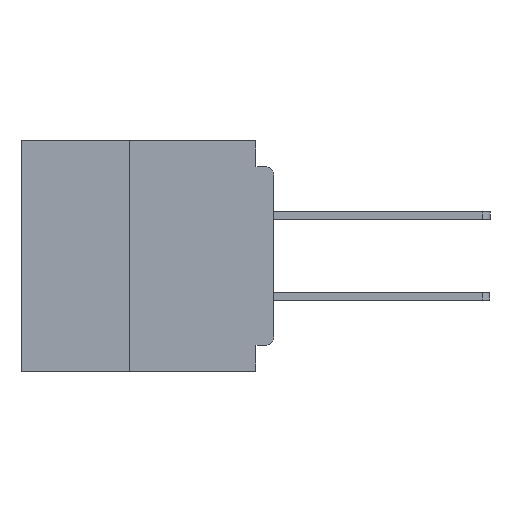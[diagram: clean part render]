
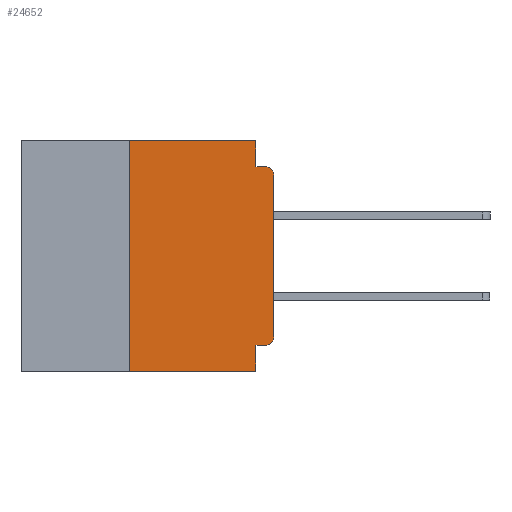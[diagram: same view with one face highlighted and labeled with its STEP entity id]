
A CAD part, left-side view. The second image highlights one B-rep face of the part: STEP entity #24652.
In plain terms, the highlighted planar face has unit normal (-1, 0, 0).
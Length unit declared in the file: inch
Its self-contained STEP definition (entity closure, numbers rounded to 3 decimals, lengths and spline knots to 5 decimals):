
#246 = DIRECTION ( 'NONE',  ( 1., 0., 0. ) ) ;
#389 = VERTEX_POINT ( 'NONE', #29512 ) ;
#532 = DIRECTION ( 'NONE',  ( 0., -1., 0. ) ) ;
#981 = VECTOR ( 'NONE', #20700, 39.37008 ) ;
#1316 = EDGE_CURVE ( 'NONE', #37058, #41313, #4289, .T. ) ;
#1412 = CIRCLE ( 'NONE', #5003, 0.015 ) ;
#1536 = EDGE_CURVE ( 'NONE', #41313, #11030, #31400, .T. ) ;
#1601 = DIRECTION ( 'NONE',  ( 0., -1., 0. ) ) ;
#1715 = ORIENTED_EDGE ( 'NONE', *, *, #9391, .T. ) ;
#2021 = EDGE_CURVE ( 'NONE', #21195, #37058, #12373, .T. ) ;
#3536 = CARTESIAN_POINT ( 'NONE',  ( 0., 0., -0.34 ) ) ;
#3734 = VECTOR ( 'NONE', #35093, 39.37008 ) ;
#3756 = CARTESIAN_POINT ( 'NONE',  ( 0., 0.437, 0. ) ) ;
#4183 = CARTESIAN_POINT ( 'NONE',  ( 0., 0.031, 0. ) ) ;
#4289 = LINE ( 'NONE', #3756, #20391 ) ;
#4397 = ORIENTED_EDGE ( 'NONE', *, *, #21143, .F. ) ;
#4438 = ORIENTED_EDGE ( 'NONE', *, *, #1536, .F. ) ;
#4540 = LINE ( 'NONE', #16035, #37647 ) ;
#5003 = AXIS2_PLACEMENT_3D ( 'NONE', #25646, #6422, #28865 ) ;
#5277 = EDGE_CURVE ( 'NONE', #7484, #40562, #1412, .T. ) ;
#6422 = DIRECTION ( 'NONE',  ( -1., 0., 0. ) ) ;
#7373 = CARTESIAN_POINT ( 'NONE',  ( 0., 0.015, -0.355 ) ) ;
#7386 = EDGE_CURVE ( 'NONE', #22626, #389, #38320, .T. ) ;
#7484 = VERTEX_POINT ( 'NONE', #7373 ) ;
#7718 = VECTOR ( 'NONE', #35284, 39.37008 ) ;
#8778 = CARTESIAN_POINT ( 'NONE',  ( 0., 0.25, -0.4 ) ) ;
#9391 = EDGE_CURVE ( 'NONE', #21195, #23236, #4540, .T. ) ;
#9522 = LINE ( 'NONE', #33441, #981 ) ;
#9540 = VERTEX_POINT ( 'NONE', #13668 ) ;
#10210 = CARTESIAN_POINT ( 'NONE',  ( 0., 0.015, -0.06 ) ) ;
#10589 = AXIS2_PLACEMENT_3D ( 'NONE', #10210, #32616, #13464 ) ;
#11030 = VERTEX_POINT ( 'NONE', #38435 ) ;
#11376 = DIRECTION ( 'NONE',  ( 0., 0., -1. ) ) ;
#12373 = LINE ( 'NONE', #8778, #3734 ) ;
#13122 = CARTESIAN_POINT ( 'NONE',  ( 0., 0.437, 0. ) ) ;
#13329 = EDGE_LOOP ( 'NONE', ( #39182, #21131, #17987, #4438, #24217, #31023, #1715, #15568, #4397, #41383 ) ) ;
#13464 = DIRECTION ( 'NONE',  ( 0., 0., -1. ) ) ;
#13668 = CARTESIAN_POINT ( 'NONE',  ( 0., 0.031, -0.355 ) ) ;
#15568 = ORIENTED_EDGE ( 'NONE', *, *, #23719, .F. ) ;
#15617 = AXIS2_PLACEMENT_3D ( 'NONE', #13122, #246, #22793 ) ;
#15793 = DIRECTION ( 'NONE',  ( 0., 0., 1. ) ) ;
#16035 = CARTESIAN_POINT ( 'NONE',  ( 0., 0.437, -0.4 ) ) ;
#17385 = VECTOR ( 'NONE', #15793, 39.37008 ) ;
#17987 = ORIENTED_EDGE ( 'NONE', *, *, #37633, .F. ) ;
#18232 = CARTESIAN_POINT ( 'NONE',  ( 0., 0.031, -0.4 ) ) ;
#18278 = LINE ( 'NONE', #28866, #7718 ) ;
#19235 = DIRECTION ( 'NONE',  ( 0., -1., 0. ) ) ;
#19510 = PLANE ( 'NONE',  #15617 ) ;
#20391 = VECTOR ( 'NONE', #532, 39.37008 ) ;
#20700 = DIRECTION ( 'NONE',  ( 0., 0., -1. ) ) ;
#21131 = ORIENTED_EDGE ( 'NONE', *, *, #7386, .T. ) ;
#21143 = EDGE_CURVE ( 'NONE', #7484, #9540, #18278, .T. ) ;
#21195 = VERTEX_POINT ( 'NONE', #29140 ) ;
#22626 = VERTEX_POINT ( 'NONE', #37570 ) ;
#22793 = DIRECTION ( 'NONE',  ( 0., 0., -1. ) ) ;
#23236 = VERTEX_POINT ( 'NONE', #18232 ) ;
#23719 = EDGE_CURVE ( 'NONE', #9540, #23236, #9522, .T. ) ;
#24104 = CARTESIAN_POINT ( 'NONE',  ( 0., 0., -0.045 ) ) ;
#24217 = ORIENTED_EDGE ( 'NONE', *, *, #1316, .F. ) ;
#24652 = ADVANCED_FACE ( 'NONE', ( #41501 ), #19510, .F. ) ;
#25646 = CARTESIAN_POINT ( 'NONE',  ( 0., 0.015, -0.34 ) ) ;
#25733 = EDGE_CURVE ( 'NONE', #40562, #22626, #33423, .T. ) ;
#28339 = VECTOR ( 'NONE', #1601, 39.37008 ) ;
#28516 = CARTESIAN_POINT ( 'NONE',  ( 0., 0., 0. ) ) ;
#28865 = DIRECTION ( 'NONE',  ( 0., 0., -1. ) ) ;
#28866 = CARTESIAN_POINT ( 'NONE',  ( 0., 0., -0.355 ) ) ;
#29140 = CARTESIAN_POINT ( 'NONE',  ( 0., 0.25, -0.4 ) ) ;
#29348 = LINE ( 'NONE', #24104, #28339 ) ;
#29512 = CARTESIAN_POINT ( 'NONE',  ( 0., 0.015, -0.045 ) ) ;
#31023 = ORIENTED_EDGE ( 'NONE', *, *, #2021, .F. ) ;
#31084 = CARTESIAN_POINT ( 'NONE',  ( 0., 0.031, 0. ) ) ;
#31400 = LINE ( 'NONE', #31084, #37883 ) ;
#32616 = DIRECTION ( 'NONE',  ( -1., 0., 0. ) ) ;
#33330 = CARTESIAN_POINT ( 'NONE',  ( 0., 0.25, 0. ) ) ;
#33423 = LINE ( 'NONE', #28516, #17385 ) ;
#33441 = CARTESIAN_POINT ( 'NONE',  ( 0., 0.031, -0.4 ) ) ;
#35093 = DIRECTION ( 'NONE',  ( 0., 0., 1. ) ) ;
#35284 = DIRECTION ( 'NONE',  ( 0., 1., 0. ) ) ;
#37058 = VERTEX_POINT ( 'NONE', #33330 ) ;
#37570 = CARTESIAN_POINT ( 'NONE',  ( 0., 0., -0.06 ) ) ;
#37633 = EDGE_CURVE ( 'NONE', #11030, #389, #29348, .T. ) ;
#37647 = VECTOR ( 'NONE', #19235, 39.37008 ) ;
#37883 = VECTOR ( 'NONE', #11376, 39.37008 ) ;
#38320 = CIRCLE ( 'NONE', #10589, 0.015 ) ;
#38435 = CARTESIAN_POINT ( 'NONE',  ( 0., 0.031, -0.045 ) ) ;
#39182 = ORIENTED_EDGE ( 'NONE', *, *, #25733, .T. ) ;
#40562 = VERTEX_POINT ( 'NONE', #3536 ) ;
#41313 = VERTEX_POINT ( 'NONE', #4183 ) ;
#41383 = ORIENTED_EDGE ( 'NONE', *, *, #5277, .T. ) ;
#41501 = FACE_OUTER_BOUND ( 'NONE', #13329, .T. ) ;
